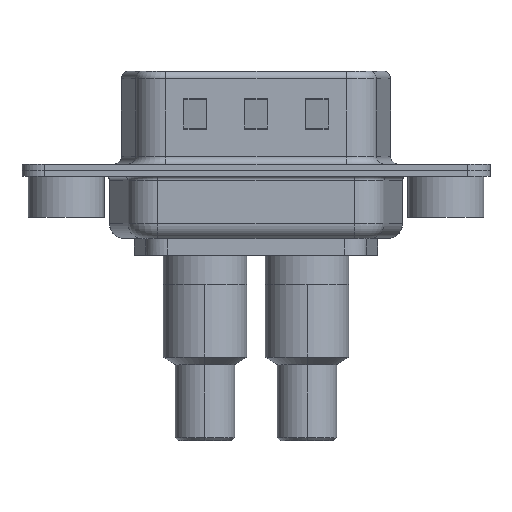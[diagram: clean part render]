
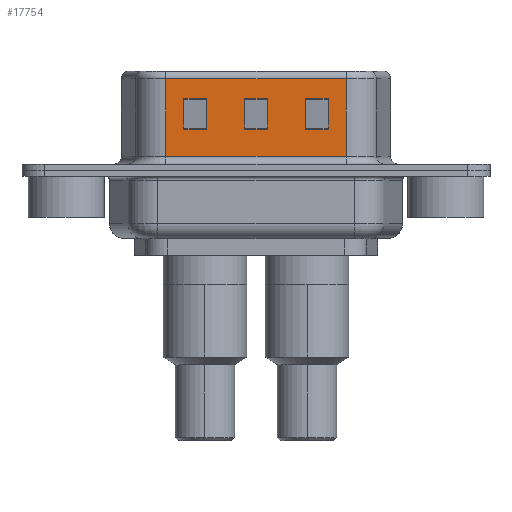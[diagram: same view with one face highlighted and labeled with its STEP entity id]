
A CAD part, front view. The second image highlights one B-rep face of the part: STEP entity #17754.
In plain terms, the highlighted planar face has unit normal (0, -1, 0).
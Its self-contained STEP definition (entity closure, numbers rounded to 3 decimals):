
#122 = EDGE_CURVE ( 'NONE', #5441, #4461, #468, .T. ) ;
#468 = LINE ( 'NONE', #8091, #15605 ) ;
#588 = VERTEX_POINT ( 'NONE', #7640 ) ;
#719 = DIRECTION ( 'NONE',  ( 0., 0., 1. ) ) ;
#766 = EDGE_CURVE ( 'NONE', #5982, #17045, #15125, .T. ) ;
#870 = EDGE_CURVE ( 'NONE', #17045, #5441, #9857, .T. ) ;
#890 = LINE ( 'NONE', #18195, #8267 ) ;
#908 = EDGE_CURVE ( 'NONE', #2953, #12041, #2112, .T. ) ;
#1114 = EDGE_LOOP ( 'NONE', ( #5159, #16752, #15148, #1722 ) ) ;
#1159 = CARTESIAN_POINT ( 'NONE',  ( 7.75, -4.58, 2.705 ) ) ;
#1253 = DIRECTION ( 'NONE',  ( 0., 0., -1. ) ) ;
#1307 = CARTESIAN_POINT ( 'NONE',  ( 18.45, -4.58, 6.02 ) ) ;
#1423 = CARTESIAN_POINT ( 'NONE',  ( 11.75, -4.58, 4.705 ) ) ;
#1443 = EDGE_CURVE ( 'NONE', #7573, #11085, #17176, .T. ) ;
#1722 = ORIENTED_EDGE ( 'NONE', *, *, #4541, .T. ) ;
#1895 = EDGE_LOOP ( 'NONE', ( #6219, #8953, #18385, #13344 ) ) ;
#2112 = LINE ( 'NONE', #4872, #16728 ) ;
#2265 = VECTOR ( 'NONE', #16479, 1000. ) ;
#2350 = CARTESIAN_POINT ( 'NONE',  ( 15.75, -4.58, 4.705 ) ) ;
#2685 = LINE ( 'NONE', #3823, #17284 ) ;
#2705 = EDGE_CURVE ( 'NONE', #12041, #588, #890, .T. ) ;
#2953 = VERTEX_POINT ( 'NONE', #5191 ) ;
#3494 = LINE ( 'NONE', #15848, #10738 ) ;
#3497 = DIRECTION ( 'NONE',  ( 0., 1., 0. ) ) ;
#3648 = EDGE_CURVE ( 'NONE', #6648, #4098, #3692, .T. ) ;
#3692 = LINE ( 'NONE', #10268, #18780 ) ;
#3823 = CARTESIAN_POINT ( 'NONE',  ( 18.45, -4.58, 6.02 ) ) ;
#4098 = VERTEX_POINT ( 'NONE', #7948 ) ;
#4235 = VECTOR ( 'NONE', #17268, 1000. ) ;
#4461 = VERTEX_POINT ( 'NONE', #18216 ) ;
#4497 = DIRECTION ( 'NONE',  ( -1., 0., 0. ) ) ;
#4541 = EDGE_CURVE ( 'NONE', #9319, #11085, #18041, .T. ) ;
#4872 = CARTESIAN_POINT ( 'NONE',  ( 11.75, -4.58, 6.52 ) ) ;
#5159 = ORIENTED_EDGE ( 'NONE', *, *, #1443, .F. ) ;
#5191 = CARTESIAN_POINT ( 'NONE',  ( 11.75, -4.58, 2.705 ) ) ;
#5285 = EDGE_CURVE ( 'NONE', #14588, #2953, #12239, .T. ) ;
#5441 = VERTEX_POINT ( 'NONE', #14454 ) ;
#5982 = VERTEX_POINT ( 'NONE', #2350 ) ;
#6202 = VERTEX_POINT ( 'NONE', #12233 ) ;
#6219 = ORIENTED_EDGE ( 'NONE', *, *, #870, .T. ) ;
#6252 = EDGE_CURVE ( 'NONE', #8208, #6202, #14040, .T. ) ;
#6254 = FACE_BOUND ( 'NONE', #16468, .T. ) ;
#6261 = CARTESIAN_POINT ( 'NONE',  ( 9.25, -4.58, 4.705 ) ) ;
#6317 = ORIENTED_EDGE ( 'NONE', *, *, #5285, .T. ) ;
#6397 = EDGE_LOOP ( 'NONE', ( #14985, #10373, #9323, #9126 ) ) ;
#6507 = VECTOR ( 'NONE', #14995, 1000. ) ;
#6600 = EDGE_CURVE ( 'NONE', #7573, #10372, #2685, .T. ) ;
#6648 = VERTEX_POINT ( 'NONE', #6261 ) ;
#6657 = DIRECTION ( 'NONE',  ( 0., 0., -1. ) ) ;
#7439 = VECTOR ( 'NONE', #14770, 1000. ) ;
#7536 = CARTESIAN_POINT ( 'NONE',  ( 14.45, -4.58, 2.705 ) ) ;
#7573 = VERTEX_POINT ( 'NONE', #1307 ) ;
#7640 = CARTESIAN_POINT ( 'NONE',  ( 13.25, -4.58, 4.705 ) ) ;
#7948 = CARTESIAN_POINT ( 'NONE',  ( 9.25, -4.58, 2.705 ) ) ;
#8091 = CARTESIAN_POINT ( 'NONE',  ( 22.45, -4.58, 2.705 ) ) ;
#8208 = VERTEX_POINT ( 'NONE', #1159 ) ;
#8267 = VECTOR ( 'NONE', #18425, 1000. ) ;
#8406 = VECTOR ( 'NONE', #10487, 1000. ) ;
#8860 = CARTESIAN_POINT ( 'NONE',  ( 18.45, -4.58, 0.9 ) ) ;
#8915 = ORIENTED_EDGE ( 'NONE', *, *, #2705, .T. ) ;
#8953 = ORIENTED_EDGE ( 'NONE', *, *, #122, .T. ) ;
#8992 = VECTOR ( 'NONE', #17984, 1000. ) ;
#9041 = DIRECTION ( 'NONE',  ( 0., 0., 1. ) ) ;
#9126 = ORIENTED_EDGE ( 'NONE', *, *, #13018, .T. ) ;
#9247 = PLANE ( 'NONE',  #13865 ) ;
#9319 = VERTEX_POINT ( 'NONE', #18605 ) ;
#9323 = ORIENTED_EDGE ( 'NONE', *, *, #6252, .T. ) ;
#9366 = ORIENTED_EDGE ( 'NONE', *, *, #908, .T. ) ;
#9716 = CARTESIAN_POINT ( 'NONE',  ( 14.45, -4.58, 4.705 ) ) ;
#9857 = LINE ( 'NONE', #18213, #17199 ) ;
#10053 = FACE_OUTER_BOUND ( 'NONE', #1114, .T. ) ;
#10177 = VECTOR ( 'NONE', #9041, 1000. ) ;
#10191 = EDGE_CURVE ( 'NONE', #10372, #9319, #18263, .T. ) ;
#10268 = CARTESIAN_POINT ( 'NONE',  ( 9.25, -4.58, 6.52 ) ) ;
#10372 = VERTEX_POINT ( 'NONE', #15142 ) ;
#10373 = ORIENTED_EDGE ( 'NONE', *, *, #18318, .T. ) ;
#10487 = DIRECTION ( 'NONE',  ( -1., 0., 0. ) ) ;
#10706 = CARTESIAN_POINT ( 'NONE',  ( 18.45, -4.58, 6.52 ) ) ;
#10738 = VECTOR ( 'NONE', #11478, 1000. ) ;
#11085 = VERTEX_POINT ( 'NONE', #8860 ) ;
#11478 = DIRECTION ( 'NONE',  ( 0., 0., -1. ) ) ;
#11879 = DIRECTION ( 'NONE',  ( -1., 0., 0. ) ) ;
#12041 = VERTEX_POINT ( 'NONE', #1423 ) ;
#12233 = CARTESIAN_POINT ( 'NONE',  ( 7.75, -4.58, 4.705 ) ) ;
#12239 = LINE ( 'NONE', #14438, #8406 ) ;
#12401 = LINE ( 'NONE', #9716, #4235 ) ;
#12731 = CARTESIAN_POINT ( 'NONE',  ( 15.75, -4.58, 6.52 ) ) ;
#12889 = LINE ( 'NONE', #12731, #8992 ) ;
#12910 = EDGE_CURVE ( 'NONE', #4461, #5982, #12889, .T. ) ;
#12968 = CARTESIAN_POINT ( 'NONE',  ( 7.75, -4.58, 6.52 ) ) ;
#13018 = EDGE_CURVE ( 'NONE', #6202, #6648, #12401, .T. ) ;
#13183 = VECTOR ( 'NONE', #18518, 1000. ) ;
#13344 = ORIENTED_EDGE ( 'NONE', *, *, #766, .T. ) ;
#13651 = DIRECTION ( 'NONE',  ( 0., 0., 1. ) ) ;
#13800 = CARTESIAN_POINT ( 'NONE',  ( 17.25, -4.58, 4.705 ) ) ;
#13865 = AXIS2_PLACEMENT_3D ( 'NONE', #10706, #3497, #13651 ) ;
#13920 = FACE_BOUND ( 'NONE', #1895, .T. ) ;
#14040 = LINE ( 'NONE', #12968, #10177 ) ;
#14415 = ORIENTED_EDGE ( 'NONE', *, *, #17356, .T. ) ;
#14438 = CARTESIAN_POINT ( 'NONE',  ( 18.45, -4.58, 2.705 ) ) ;
#14454 = CARTESIAN_POINT ( 'NONE',  ( 17.25, -4.58, 2.705 ) ) ;
#14588 = VERTEX_POINT ( 'NONE', #15115 ) ;
#14770 = DIRECTION ( 'NONE',  ( 1., 0., 0. ) ) ;
#14821 = LINE ( 'NONE', #7536, #17823 ) ;
#14958 = CARTESIAN_POINT ( 'NONE',  ( 22.45, -4.58, 4.705 ) ) ;
#14985 = ORIENTED_EDGE ( 'NONE', *, *, #3648, .T. ) ;
#14995 = DIRECTION ( 'NONE',  ( 0., 0., -1. ) ) ;
#15115 = CARTESIAN_POINT ( 'NONE',  ( 13.25, -4.58, 2.705 ) ) ;
#15125 = LINE ( 'NONE', #14958, #7439 ) ;
#15142 = CARTESIAN_POINT ( 'NONE',  ( 6.55, -4.58, 6.02 ) ) ;
#15148 = ORIENTED_EDGE ( 'NONE', *, *, #10191, .T. ) ;
#15247 = CARTESIAN_POINT ( 'NONE',  ( 18.45, -4.58, 0.9 ) ) ;
#15605 = VECTOR ( 'NONE', #11879, 1000. ) ;
#15848 = CARTESIAN_POINT ( 'NONE',  ( 13.25, -4.58, 6.52 ) ) ;
#16468 = EDGE_LOOP ( 'NONE', ( #8915, #14415, #6317, #9366 ) ) ;
#16479 = DIRECTION ( 'NONE',  ( 0., 0., -1. ) ) ;
#16492 = CARTESIAN_POINT ( 'NONE',  ( 6.55, -4.58, 6.52 ) ) ;
#16728 = VECTOR ( 'NONE', #719, 1000. ) ;
#16752 = ORIENTED_EDGE ( 'NONE', *, *, #6600, .T. ) ;
#17045 = VERTEX_POINT ( 'NONE', #13800 ) ;
#17176 = LINE ( 'NONE', #17809, #6507 ) ;
#17199 = VECTOR ( 'NONE', #1253, 1000. ) ;
#17268 = DIRECTION ( 'NONE',  ( 1., 0., 0. ) ) ;
#17284 = VECTOR ( 'NONE', #4497, 1000. ) ;
#17356 = EDGE_CURVE ( 'NONE', #588, #14588, #3494, .T. ) ;
#17384 = FACE_BOUND ( 'NONE', #6397, .T. ) ;
#17688 = DIRECTION ( 'NONE',  ( -1., 0., 0. ) ) ;
#17754 = ADVANCED_FACE ( 'NONE', ( #17384, #13920, #6254, #10053 ), #9247, .F. ) ;
#17809 = CARTESIAN_POINT ( 'NONE',  ( 18.45, -4.58, 6.52 ) ) ;
#17823 = VECTOR ( 'NONE', #17688, 1000. ) ;
#17984 = DIRECTION ( 'NONE',  ( 0., 0., 1. ) ) ;
#18041 = LINE ( 'NONE', #15247, #13183 ) ;
#18195 = CARTESIAN_POINT ( 'NONE',  ( 18.45, -4.58, 4.705 ) ) ;
#18213 = CARTESIAN_POINT ( 'NONE',  ( 17.25, -4.58, 6.52 ) ) ;
#18216 = CARTESIAN_POINT ( 'NONE',  ( 15.75, -4.58, 2.705 ) ) ;
#18263 = LINE ( 'NONE', #16492, #2265 ) ;
#18318 = EDGE_CURVE ( 'NONE', #4098, #8208, #14821, .T. ) ;
#18385 = ORIENTED_EDGE ( 'NONE', *, *, #12910, .T. ) ;
#18425 = DIRECTION ( 'NONE',  ( 1., 0., 0. ) ) ;
#18518 = DIRECTION ( 'NONE',  ( 1., 0., 0. ) ) ;
#18605 = CARTESIAN_POINT ( 'NONE',  ( 6.55, -4.58, 0.9 ) ) ;
#18780 = VECTOR ( 'NONE', #6657, 1000. ) ;
